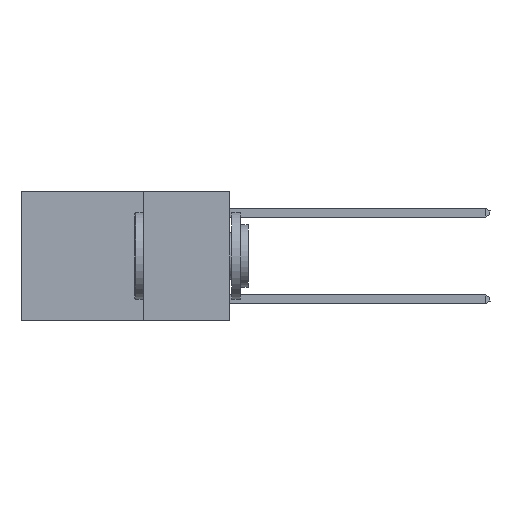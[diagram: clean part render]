
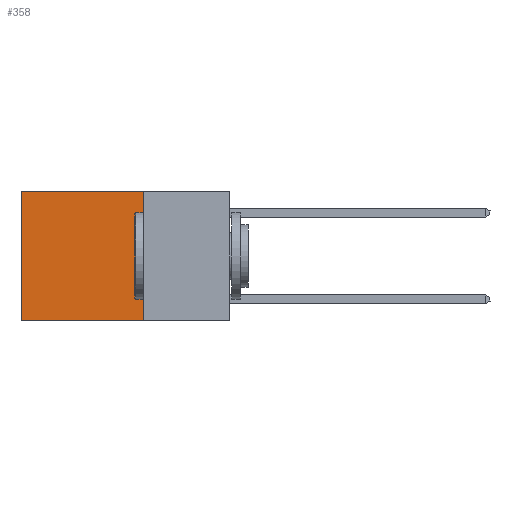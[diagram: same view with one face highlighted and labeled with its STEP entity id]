
A CAD part, left-side view. The second image highlights one B-rep face of the part: STEP entity #358.
In plain terms, the highlighted planar face has unit normal (-1, 0, 0).
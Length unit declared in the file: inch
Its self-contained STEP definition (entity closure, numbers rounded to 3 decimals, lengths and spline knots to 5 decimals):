
#358 = ADVANCED_FACE ( 'NONE', ( #7167 ), #16104, .F. ) ;
#2666 = VECTOR ( 'NONE', #5072, 39.37008 ) ;
#2751 = DIRECTION ( 'NONE',  ( 0., 0., -1. ) ) ;
#3445 = ORIENTED_EDGE ( 'NONE', *, *, #17221, .F. ) ;
#4524 = VERTEX_POINT ( 'NONE', #19583 ) ;
#4964 = CARTESIAN_POINT ( 'NONE',  ( 0.2625, 0.25, 0. ) ) ;
#5036 = EDGE_CURVE ( 'NONE', #25599, #4524, #26600, .T. ) ;
#5072 = DIRECTION ( 'NONE',  ( 0., 0., -1. ) ) ;
#5759 = EDGE_CURVE ( 'NONE', #28879, #22152, #16641, .T. ) ;
#6261 = VECTOR ( 'NONE', #16428, 39.37008 ) ;
#7167 = FACE_OUTER_BOUND ( 'NONE', #24210, .T. ) ;
#7497 = LINE ( 'NONE', #12042, #6261 ) ;
#12042 = CARTESIAN_POINT ( 'NONE',  ( 0.2625, 0.25, 0. ) ) ;
#12347 = VECTOR ( 'NONE', #20542, 39.37008 ) ;
#12770 = LINE ( 'NONE', #28529, #12347 ) ;
#13903 = DIRECTION ( 'NONE',  ( 1., 0., 0. ) ) ;
#15660 = EDGE_CURVE ( 'NONE', #25599, #28879, #7497, .T. ) ;
#16104 = PLANE ( 'NONE',  #24458 ) ;
#16428 = DIRECTION ( 'NONE',  ( 0., 1., 0. ) ) ;
#16641 = LINE ( 'NONE', #18566, #2666 ) ;
#16898 = ORIENTED_EDGE ( 'NONE', *, *, #5759, .T. ) ;
#17221 = EDGE_CURVE ( 'NONE', #4524, #22152, #12770, .T. ) ;
#18566 = CARTESIAN_POINT ( 'NONE',  ( 0.2625, 0.6, 0. ) ) ;
#19583 = CARTESIAN_POINT ( 'NONE',  ( 0.2625, 0.25, -0.37 ) ) ;
#20542 = DIRECTION ( 'NONE',  ( 0., 1., 0. ) ) ;
#21852 = CARTESIAN_POINT ( 'NONE',  ( 0.2625, 0.25, 0. ) ) ;
#22152 = VERTEX_POINT ( 'NONE', #28912 ) ;
#22176 = DIRECTION ( 'NONE',  ( 0., 0., -1. ) ) ;
#22319 = ORIENTED_EDGE ( 'NONE', *, *, #15660, .T. ) ;
#23573 = CARTESIAN_POINT ( 'NONE',  ( 0.2625, 0.6, 0. ) ) ;
#23805 = CARTESIAN_POINT ( 'NONE',  ( 0.2625, 0.25, 0. ) ) ;
#24210 = EDGE_LOOP ( 'NONE', ( #16898, #3445, #26790, #22319 ) ) ;
#24458 = AXIS2_PLACEMENT_3D ( 'NONE', #4964, #13903, #2751 ) ;
#25599 = VERTEX_POINT ( 'NONE', #21852 ) ;
#26600 = LINE ( 'NONE', #23805, #26988 ) ;
#26790 = ORIENTED_EDGE ( 'NONE', *, *, #5036, .F. ) ;
#26988 = VECTOR ( 'NONE', #22176, 39.37008 ) ;
#28529 = CARTESIAN_POINT ( 'NONE',  ( 0.2625, 0.25, -0.37 ) ) ;
#28879 = VERTEX_POINT ( 'NONE', #23573 ) ;
#28912 = CARTESIAN_POINT ( 'NONE',  ( 0.2625, 0.6, -0.37 ) ) ;
